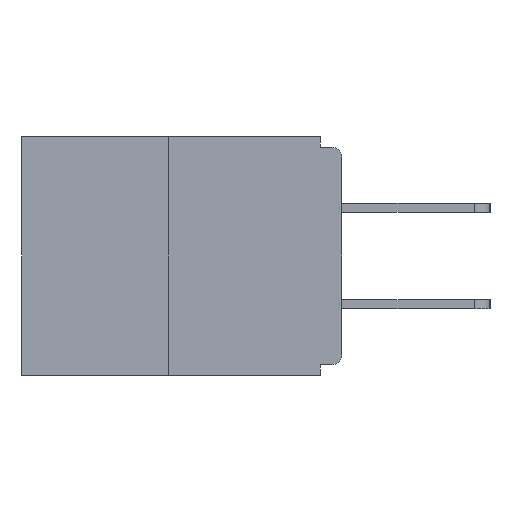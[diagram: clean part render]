
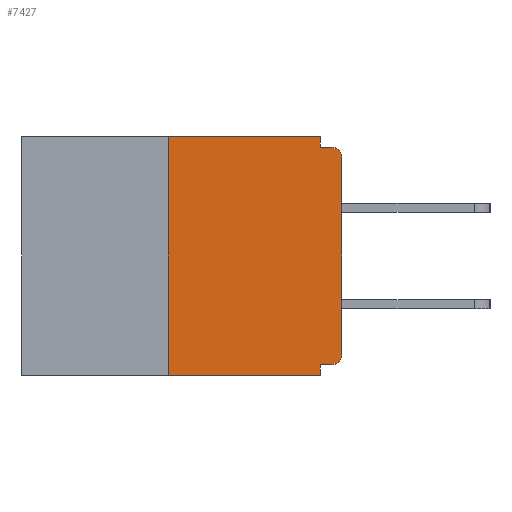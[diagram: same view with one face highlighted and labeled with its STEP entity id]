
A CAD part, left-side view. The second image highlights one B-rep face of the part: STEP entity #7427.
In plain terms, the highlighted planar face has unit normal (-1, 0, 0).
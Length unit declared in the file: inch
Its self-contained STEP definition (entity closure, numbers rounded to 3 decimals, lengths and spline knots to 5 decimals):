
#273 = DIRECTION ( 'NONE',  ( 1., 0., 0. ) ) ;
#1108 = AXIS2_PLACEMENT_3D ( 'NONE', #5328, #5531, #7863 ) ;
#1561 = CARTESIAN_POINT ( 'NONE',  ( 0., 0.031, -0.343 ) ) ;
#1673 = EDGE_CURVE ( 'NONE', #17732, #19318, #22656, .T. ) ;
#2060 = CARTESIAN_POINT ( 'NONE',  ( 0., 0.25, -0.343 ) ) ;
#2504 = ORIENTED_EDGE ( 'NONE', *, *, #1673, .F. ) ;
#2533 = VERTEX_POINT ( 'NONE', #21753 ) ;
#2640 = FACE_OUTER_BOUND ( 'NONE', #22491, .T. ) ;
#2666 = ORIENTED_EDGE ( 'NONE', *, *, #19247, .F. ) ;
#2729 = CARTESIAN_POINT ( 'NONE',  ( 0., 0., 0. ) ) ;
#2734 = CARTESIAN_POINT ( 'NONE',  ( 0., 0.031, -0.343 ) ) ;
#3185 = ORIENTED_EDGE ( 'NONE', *, *, #7554, .T. ) ;
#3521 = CARTESIAN_POINT ( 'NONE',  ( 0., 0.25, 0. ) ) ;
#3599 = LINE ( 'NONE', #19922, #21902 ) ;
#3646 = ORIENTED_EDGE ( 'NONE', *, *, #19834, .F. ) ;
#4278 = LINE ( 'NONE', #2729, #25872 ) ;
#5328 = CARTESIAN_POINT ( 'NONE',  ( 0., 0.015, -0.03 ) ) ;
#5531 = DIRECTION ( 'NONE',  ( -1., 0., 0. ) ) ;
#5799 = EDGE_CURVE ( 'NONE', #27701, #19518, #7814, .T. ) ;
#6007 = DIRECTION ( 'NONE',  ( -1., 0., 0. ) ) ;
#6032 = CARTESIAN_POINT ( 'NONE',  ( 0., 0.031, 0. ) ) ;
#7175 = LINE ( 'NONE', #19527, #29170 ) ;
#7323 = VERTEX_POINT ( 'NONE', #8068 ) ;
#7427 = ADVANCED_FACE ( 'NONE', ( #2640 ), #28329, .F. ) ;
#7554 = EDGE_CURVE ( 'NONE', #2533, #7323, #18005, .T. ) ;
#7814 = LINE ( 'NONE', #1561, #16599 ) ;
#7863 = DIRECTION ( 'NONE',  ( 0., 0., -1. ) ) ;
#8068 = CARTESIAN_POINT ( 'NONE',  ( 0., 0., -0.313 ) ) ;
#8096 = VERTEX_POINT ( 'NONE', #19694 ) ;
#8237 = CARTESIAN_POINT ( 'NONE',  ( 0., 0.015, -0.313 ) ) ;
#9563 = EDGE_CURVE ( 'NONE', #30004, #8096, #15674, .T. ) ;
#9661 = ORIENTED_EDGE ( 'NONE', *, *, #16234, .T. ) ;
#10382 = ORIENTED_EDGE ( 'NONE', *, *, #19188, .T. ) ;
#10518 = CARTESIAN_POINT ( 'NONE',  ( 0., 0., -0.328 ) ) ;
#11249 = DIRECTION ( 'NONE',  ( 0., 1., 0. ) ) ;
#12301 = VERTEX_POINT ( 'NONE', #16121 ) ;
#12997 = LINE ( 'NONE', #30399, #21774 ) ;
#13409 = ORIENTED_EDGE ( 'NONE', *, *, #24500, .T. ) ;
#13935 = LINE ( 'NONE', #10518, #22351 ) ;
#14311 = CARTESIAN_POINT ( 'NONE',  ( 0., 0.46, 0. ) ) ;
#15319 = VECTOR ( 'NONE', #29589, 39.37008 ) ;
#15674 = LINE ( 'NONE', #3521, #26281 ) ;
#16121 = CARTESIAN_POINT ( 'NONE',  ( 0., 0., -0.03 ) ) ;
#16234 = EDGE_CURVE ( 'NONE', #30004, #19518, #3599, .T. ) ;
#16599 = VECTOR ( 'NONE', #20208, 39.37008 ) ;
#17732 = VERTEX_POINT ( 'NONE', #18721 ) ;
#17860 = DIRECTION ( 'NONE',  ( 0., -1., 0. ) ) ;
#18005 = CIRCLE ( 'NONE', #29248, 0.015 ) ;
#18256 = AXIS2_PLACEMENT_3D ( 'NONE', #14311, #273, #21457 ) ;
#18721 = CARTESIAN_POINT ( 'NONE',  ( 0., 0.031, 0. ) ) ;
#19188 = EDGE_CURVE ( 'NONE', #7323, #12301, #4278, .T. ) ;
#19247 = EDGE_CURVE ( 'NONE', #8096, #17732, #7175, .T. ) ;
#19318 = VERTEX_POINT ( 'NONE', #19419 ) ;
#19342 = ORIENTED_EDGE ( 'NONE', *, *, #23247, .F. ) ;
#19419 = CARTESIAN_POINT ( 'NONE',  ( 0., 0.031, -0.015 ) ) ;
#19518 = VERTEX_POINT ( 'NONE', #2734 ) ;
#19527 = CARTESIAN_POINT ( 'NONE',  ( 0., 0.46, 0. ) ) ;
#19694 = CARTESIAN_POINT ( 'NONE',  ( 0., 0.25, 0. ) ) ;
#19834 = EDGE_CURVE ( 'NONE', #19318, #23226, #12997, .T. ) ;
#19922 = CARTESIAN_POINT ( 'NONE',  ( 0., 0.46, -0.343 ) ) ;
#20208 = DIRECTION ( 'NONE',  ( 0., 0., -1. ) ) ;
#20833 = DIRECTION ( 'NONE',  ( 0., -1., 0. ) ) ;
#21457 = DIRECTION ( 'NONE',  ( 0., 0., -1. ) ) ;
#21753 = CARTESIAN_POINT ( 'NONE',  ( 0., 0.015, -0.328 ) ) ;
#21755 = DIRECTION ( 'NONE',  ( 0., -1., 0. ) ) ;
#21774 = VECTOR ( 'NONE', #20833, 39.37008 ) ;
#21902 = VECTOR ( 'NONE', #17860, 39.37008 ) ;
#22351 = VECTOR ( 'NONE', #11249, 39.37008 ) ;
#22491 = EDGE_LOOP ( 'NONE', ( #2666, #27001, #9661, #28045, #19342, #3185, #10382, #13409, #3646, #2504 ) ) ;
#22656 = LINE ( 'NONE', #6032, #15319 ) ;
#23226 = VERTEX_POINT ( 'NONE', #25183 ) ;
#23247 = EDGE_CURVE ( 'NONE', #2533, #27701, #13935, .T. ) ;
#23821 = CARTESIAN_POINT ( 'NONE',  ( 0., 0.031, -0.328 ) ) ;
#23912 = DIRECTION ( 'NONE',  ( 0., 0., 1. ) ) ;
#24288 = DIRECTION ( 'NONE',  ( 0., 0., 1. ) ) ;
#24500 = EDGE_CURVE ( 'NONE', #12301, #23226, #29273, .T. ) ;
#24623 = DIRECTION ( 'NONE',  ( 0., 0., -1. ) ) ;
#25183 = CARTESIAN_POINT ( 'NONE',  ( 0., 0.015, -0.015 ) ) ;
#25872 = VECTOR ( 'NONE', #23912, 39.37008 ) ;
#26281 = VECTOR ( 'NONE', #24288, 39.37008 ) ;
#27001 = ORIENTED_EDGE ( 'NONE', *, *, #9563, .F. ) ;
#27701 = VERTEX_POINT ( 'NONE', #23821 ) ;
#28045 = ORIENTED_EDGE ( 'NONE', *, *, #5799, .F. ) ;
#28329 = PLANE ( 'NONE',  #18256 ) ;
#29170 = VECTOR ( 'NONE', #21755, 39.37008 ) ;
#29248 = AXIS2_PLACEMENT_3D ( 'NONE', #8237, #6007, #24623 ) ;
#29273 = CIRCLE ( 'NONE', #1108, 0.015 ) ;
#29589 = DIRECTION ( 'NONE',  ( 0., 0., -1. ) ) ;
#30004 = VERTEX_POINT ( 'NONE', #2060 ) ;
#30399 = CARTESIAN_POINT ( 'NONE',  ( 0., 0., -0.015 ) ) ;
